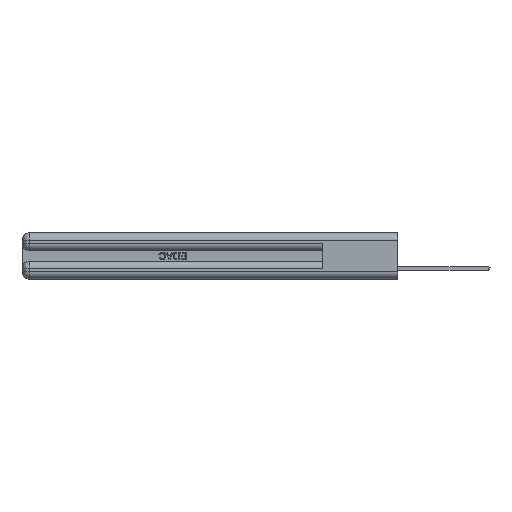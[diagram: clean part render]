
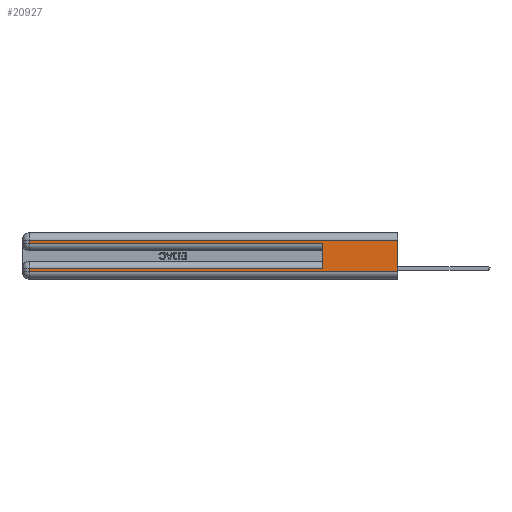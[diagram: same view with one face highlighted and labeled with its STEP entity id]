
A CAD part, left-side view. The second image highlights one B-rep face of the part: STEP entity #20927.
In plain terms, the highlighted planar face has unit normal (-1, 0, 0).
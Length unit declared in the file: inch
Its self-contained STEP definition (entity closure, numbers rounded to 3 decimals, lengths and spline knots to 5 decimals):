
#78 = ORIENTED_EDGE ( 'NONE', *, *, #27103, .T. ) ;
#1664 = CARTESIAN_POINT ( 'NONE',  ( 0., 0., 0.06 ) ) ;
#1703 = EDGE_CURVE ( 'NONE', #17702, #29728, #43387, .T. ) ;
#1969 = EDGE_CURVE ( 'NONE', #17702, #37320, #2787, .T. ) ;
#2664 = LINE ( 'NONE', #37682, #40391 ) ;
#2787 = LINE ( 'NONE', #14620, #37043 ) ;
#3581 = ORIENTED_EDGE ( 'NONE', *, *, #17620, .T. ) ;
#6110 = CARTESIAN_POINT ( 'NONE',  ( 0., 0., 0.37 ) ) ;
#6644 = LINE ( 'NONE', #14159, #25927 ) ;
#8093 = CARTESIAN_POINT ( 'NONE',  ( 0., 2.94, 0.37 ) ) ;
#8156 = ORIENTED_EDGE ( 'NONE', *, *, #19037, .T. ) ;
#8558 = ORIENTED_EDGE ( 'NONE', *, *, #1969, .T. ) ;
#9259 = DIRECTION ( 'NONE',  ( 1., 0., 0. ) ) ;
#9576 = VERTEX_POINT ( 'NONE', #34298 ) ;
#9649 = VECTOR ( 'NONE', #17880, 39.37008 ) ;
#9704 = CARTESIAN_POINT ( 'NONE',  ( 0., 2.94, 0.06 ) ) ;
#11022 = LINE ( 'NONE', #1664, #13294 ) ;
#12151 = VECTOR ( 'NONE', #31667, 39.37008 ) ;
#12348 = CARTESIAN_POINT ( 'NONE',  ( 0., 2.94, 0.31 ) ) ;
#12681 = EDGE_CURVE ( 'NONE', #9576, #30025, #28115, .T. ) ;
#13294 = VECTOR ( 'NONE', #27001, 39.37008 ) ;
#13755 = VECTOR ( 'NONE', #26809, 39.37008 ) ;
#14159 = CARTESIAN_POINT ( 'NONE',  ( 0., 2.94, 0.37 ) ) ;
#14620 = CARTESIAN_POINT ( 'NONE',  ( 0., 0., 0.085 ) ) ;
#15369 = LINE ( 'NONE', #8093, #13755 ) ;
#16556 = AXIS2_PLACEMENT_3D ( 'NONE', #6110, #9259, #16741 ) ;
#16741 = DIRECTION ( 'NONE',  ( 0., 0., -1. ) ) ;
#17336 = DIRECTION ( 'NONE',  ( 0., 1., 0. ) ) ;
#17620 = EDGE_CURVE ( 'NONE', #37320, #18011, #6644, .T. ) ;
#17702 = VERTEX_POINT ( 'NONE', #43005 ) ;
#17880 = DIRECTION ( 'NONE',  ( 0., 0., 1. ) ) ;
#18011 = VERTEX_POINT ( 'NONE', #9704 ) ;
#19037 = EDGE_CURVE ( 'NONE', #9576, #21187, #24087, .T. ) ;
#20927 = ADVANCED_FACE ( 'NONE', ( #22857 ), #35120, .F. ) ;
#21187 = VERTEX_POINT ( 'NONE', #12348 ) ;
#22857 = FACE_OUTER_BOUND ( 'NONE', #23151, .T. ) ;
#22974 = ORIENTED_EDGE ( 'NONE', *, *, #39075, .T. ) ;
#23151 = EDGE_LOOP ( 'NONE', ( #26255, #8156, #22974, #36041, #30852, #8558, #3581, #78 ) ) ;
#24087 = LINE ( 'NONE', #39089, #30258 ) ;
#24442 = EDGE_CURVE ( 'NONE', #30188, #29728, #2664, .T. ) ;
#25017 = CARTESIAN_POINT ( 'NONE',  ( 0., 0.6, 0.145 ) ) ;
#25927 = VECTOR ( 'NONE', #28975, 39.37008 ) ;
#26255 = ORIENTED_EDGE ( 'NONE', *, *, #12681, .F. ) ;
#26809 = DIRECTION ( 'NONE',  ( 0., 0., -1. ) ) ;
#27001 = DIRECTION ( 'NONE',  ( 0., -1., 0. ) ) ;
#27103 = EDGE_CURVE ( 'NONE', #18011, #30025, #11022, .T. ) ;
#27158 = CARTESIAN_POINT ( 'NONE',  ( 0., 2.94, 0.285 ) ) ;
#27308 = CARTESIAN_POINT ( 'NONE',  ( 0., 2.94, 0.085 ) ) ;
#27387 = CARTESIAN_POINT ( 'NONE',  ( 0., 0., 0.06 ) ) ;
#28115 = LINE ( 'NONE', #42121, #12151 ) ;
#28975 = DIRECTION ( 'NONE',  ( 0., 0., -1. ) ) ;
#29728 = VERTEX_POINT ( 'NONE', #41752 ) ;
#30025 = VERTEX_POINT ( 'NONE', #27387 ) ;
#30188 = VERTEX_POINT ( 'NONE', #27158 ) ;
#30258 = VECTOR ( 'NONE', #17336, 39.37008 ) ;
#30852 = ORIENTED_EDGE ( 'NONE', *, *, #1703, .F. ) ;
#31667 = DIRECTION ( 'NONE',  ( 0., 0., -1. ) ) ;
#34298 = CARTESIAN_POINT ( 'NONE',  ( 0., 0., 0.31 ) ) ;
#35120 = PLANE ( 'NONE',  #16556 ) ;
#36041 = ORIENTED_EDGE ( 'NONE', *, *, #24442, .T. ) ;
#37043 = VECTOR ( 'NONE', #40203, 39.37008 ) ;
#37320 = VERTEX_POINT ( 'NONE', #27308 ) ;
#37682 = CARTESIAN_POINT ( 'NONE',  ( 0., 0., 0.285 ) ) ;
#39075 = EDGE_CURVE ( 'NONE', #21187, #30188, #15369, .T. ) ;
#39089 = CARTESIAN_POINT ( 'NONE',  ( 0., 0., 0.31 ) ) ;
#40203 = DIRECTION ( 'NONE',  ( 0., 1., 0. ) ) ;
#40391 = VECTOR ( 'NONE', #41532, 39.37008 ) ;
#41532 = DIRECTION ( 'NONE',  ( 0., -1., 0. ) ) ;
#41752 = CARTESIAN_POINT ( 'NONE',  ( 0., 0.6, 0.285 ) ) ;
#42121 = CARTESIAN_POINT ( 'NONE',  ( 0., 0., 0.37 ) ) ;
#43005 = CARTESIAN_POINT ( 'NONE',  ( 0., 0.6, 0.085 ) ) ;
#43387 = LINE ( 'NONE', #25017, #9649 ) ;
